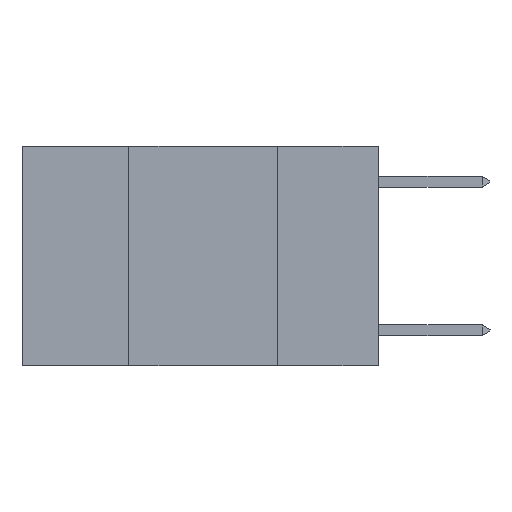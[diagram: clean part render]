
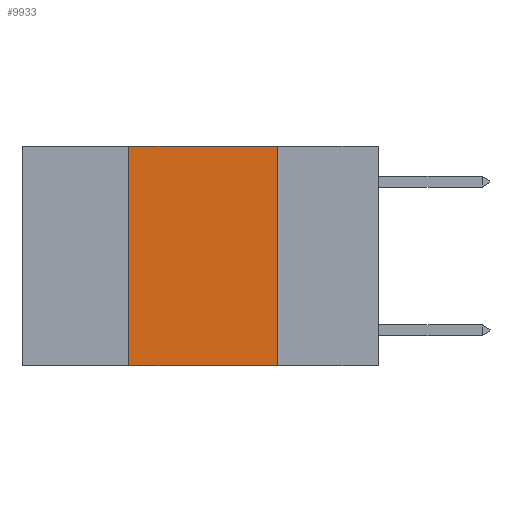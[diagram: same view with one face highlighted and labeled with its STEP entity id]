
A CAD part, left-side view. The second image highlights one B-rep face of the part: STEP entity #9933.
In plain terms, the highlighted planar face has unit normal (-1, 0, 0).
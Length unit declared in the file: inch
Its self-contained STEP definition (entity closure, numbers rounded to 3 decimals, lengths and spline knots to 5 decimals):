
#424 = VERTEX_POINT ( 'NONE', #2378 ) ;
#470 = VECTOR ( 'NONE', #15190, 39.37008 ) ;
#485 = ORIENTED_EDGE ( 'NONE', *, *, #8887, .F. ) ;
#493 = DIRECTION ( 'NONE',  ( 0., 0., -1. ) ) ;
#2378 = CARTESIAN_POINT ( 'NONE',  ( 0., 0.17, -0.37 ) ) ;
#2394 = FACE_OUTER_BOUND ( 'NONE', #14334, .T. ) ;
#2528 = VECTOR ( 'NONE', #493, 39.37008 ) ;
#3433 = ORIENTED_EDGE ( 'NONE', *, *, #6756, .F. ) ;
#3842 = CARTESIAN_POINT ( 'NONE',  ( 0., 0.6, 0. ) ) ;
#4721 = LINE ( 'NONE', #8935, #2528 ) ;
#5016 = VERTEX_POINT ( 'NONE', #10595 ) ;
#6111 = LINE ( 'NONE', #8644, #17432 ) ;
#6756 = EDGE_CURVE ( 'NONE', #5016, #11873, #6111, .T. ) ;
#8427 = VERTEX_POINT ( 'NONE', #11469 ) ;
#8644 = CARTESIAN_POINT ( 'NONE',  ( 0., 0.6, 0. ) ) ;
#8881 = DIRECTION ( 'NONE',  ( 0., 0., 1. ) ) ;
#8887 = EDGE_CURVE ( 'NONE', #8427, #5016, #17240, .T. ) ;
#8935 = CARTESIAN_POINT ( 'NONE',  ( 0., 0.17, 0. ) ) ;
#8970 = CARTESIAN_POINT ( 'NONE',  ( 0., 0.42, 0. ) ) ;
#8995 = ORIENTED_EDGE ( 'NONE', *, *, #14438, .T. ) ;
#9016 = PLANE ( 'NONE',  #16784 ) ;
#9277 = DIRECTION ( 'NONE',  ( 0., 0., -1. ) ) ;
#9591 = CARTESIAN_POINT ( 'NONE',  ( 0., 0.6, -0.37 ) ) ;
#9933 = ADVANCED_FACE ( 'NONE', ( #2394 ), #9016, .F. ) ;
#10217 = ORIENTED_EDGE ( 'NONE', *, *, #13833, .F. ) ;
#10595 = CARTESIAN_POINT ( 'NONE',  ( 0., 0.42, 0. ) ) ;
#11095 = VECTOR ( 'NONE', #8881, 39.37008 ) ;
#11469 = CARTESIAN_POINT ( 'NONE',  ( 0., 0.42, -0.37 ) ) ;
#11670 = DIRECTION ( 'NONE',  ( 1., 0., 0. ) ) ;
#11873 = VERTEX_POINT ( 'NONE', #13758 ) ;
#13758 = CARTESIAN_POINT ( 'NONE',  ( 0., 0.17, 0. ) ) ;
#13833 = EDGE_CURVE ( 'NONE', #11873, #424, #4721, .T. ) ;
#14334 = EDGE_LOOP ( 'NONE', ( #10217, #3433, #485, #8995 ) ) ;
#14438 = EDGE_CURVE ( 'NONE', #8427, #424, #15274, .T. ) ;
#15190 = DIRECTION ( 'NONE',  ( 0., -1., 0. ) ) ;
#15274 = LINE ( 'NONE', #9591, #470 ) ;
#15639 = DIRECTION ( 'NONE',  ( 0., -1., 0. ) ) ;
#16784 = AXIS2_PLACEMENT_3D ( 'NONE', #3842, #11670, #9277 ) ;
#17240 = LINE ( 'NONE', #8970, #11095 ) ;
#17432 = VECTOR ( 'NONE', #15639, 39.37008 ) ;
